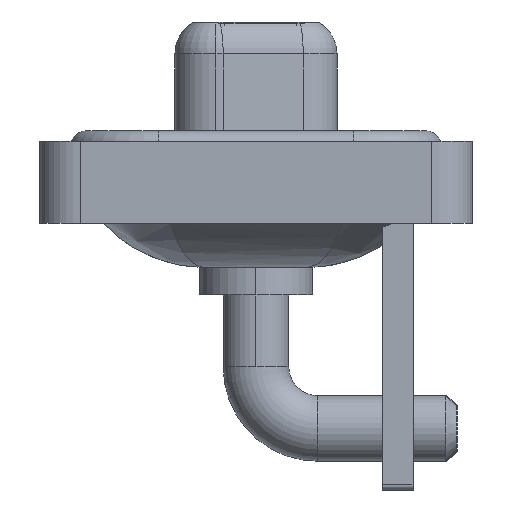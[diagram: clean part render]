
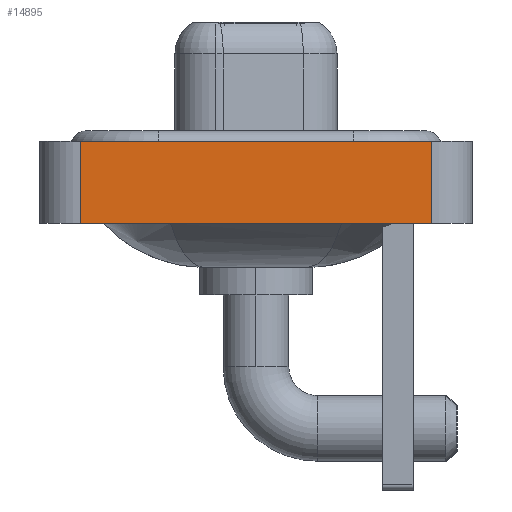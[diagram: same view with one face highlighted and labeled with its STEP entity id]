
A CAD part, left-side view. The second image highlights one B-rep face of the part: STEP entity #14895.
In plain terms, the highlighted planar face has unit normal (-1, 0, 0).
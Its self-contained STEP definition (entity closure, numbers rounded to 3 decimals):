
#269 = PLANE ( 'NONE',  #10991 ) ;
#1184 = CARTESIAN_POINT ( 'NONE',  ( -7.3, 8.55, 0.4 ) ) ;
#1542 = LINE ( 'NONE', #5696, #2603 ) ;
#1576 = FACE_OUTER_BOUND ( 'NONE', #9995, .T. ) ;
#2028 = DIRECTION ( 'NONE',  ( 0., 0., 1. ) ) ;
#2114 = LINE ( 'NONE', #4808, #5579 ) ;
#2166 = CARTESIAN_POINT ( 'NONE',  ( -7.3, 8.55, -3.6 ) ) ;
#2268 = VECTOR ( 'NONE', #8036, 1000. ) ;
#2603 = VECTOR ( 'NONE', #7179, 1000. ) ;
#3267 = VERTEX_POINT ( 'NONE', #12159 ) ;
#4808 = CARTESIAN_POINT ( 'NONE',  ( -7.3, -8.55, -3.6 ) ) ;
#4841 = EDGE_CURVE ( 'NONE', #3267, #5749, #1542, .T. ) ;
#4946 = LINE ( 'NONE', #2166, #10167 ) ;
#5166 = ORIENTED_EDGE ( 'NONE', *, *, #12474, .F. ) ;
#5504 = EDGE_CURVE ( 'NONE', #5749, #12320, #2114, .T. ) ;
#5579 = VECTOR ( 'NONE', #2028, 1000. ) ;
#5696 = CARTESIAN_POINT ( 'NONE',  ( -7.3, -8.55, -3.6 ) ) ;
#5749 = VERTEX_POINT ( 'NONE', #16625 ) ;
#5924 = DIRECTION ( 'NONE',  ( -1., 0., 0. ) ) ;
#7179 = DIRECTION ( 'NONE',  ( 0., -1., 0. ) ) ;
#7554 = CARTESIAN_POINT ( 'NONE',  ( -7.3, -8.55, 0.4 ) ) ;
#8036 = DIRECTION ( 'NONE',  ( 0., -1., 0. ) ) ;
#9122 = ORIENTED_EDGE ( 'NONE', *, *, #10798, .F. ) ;
#9995 = EDGE_LOOP ( 'NONE', ( #12488, #9122, #5166, #10423 ) ) ;
#10167 = VECTOR ( 'NONE', #17870, 1000. ) ;
#10423 = ORIENTED_EDGE ( 'NONE', *, *, #4841, .T. ) ;
#10719 = CARTESIAN_POINT ( 'NONE',  ( -7.3, -8.55, 0.4 ) ) ;
#10798 = EDGE_CURVE ( 'NONE', #12910, #12320, #10810, .T. ) ;
#10810 = LINE ( 'NONE', #10719, #2268 ) ;
#10991 = AXIS2_PLACEMENT_3D ( 'NONE', #15798, #5924, #17183 ) ;
#12159 = CARTESIAN_POINT ( 'NONE',  ( -7.3, 8.55, -3.6 ) ) ;
#12320 = VERTEX_POINT ( 'NONE', #7554 ) ;
#12474 = EDGE_CURVE ( 'NONE', #3267, #12910, #4946, .T. ) ;
#12488 = ORIENTED_EDGE ( 'NONE', *, *, #5504, .T. ) ;
#12910 = VERTEX_POINT ( 'NONE', #1184 ) ;
#14895 = ADVANCED_FACE ( 'NONE', ( #1576 ), #269, .T. ) ;
#15798 = CARTESIAN_POINT ( 'NONE',  ( -7.3, -8.55, -3.6 ) ) ;
#16625 = CARTESIAN_POINT ( 'NONE',  ( -7.3, -8.55, -3.6 ) ) ;
#17183 = DIRECTION ( 'NONE',  ( 0., 0., 1. ) ) ;
#17870 = DIRECTION ( 'NONE',  ( 0., 0., 1. ) ) ;
